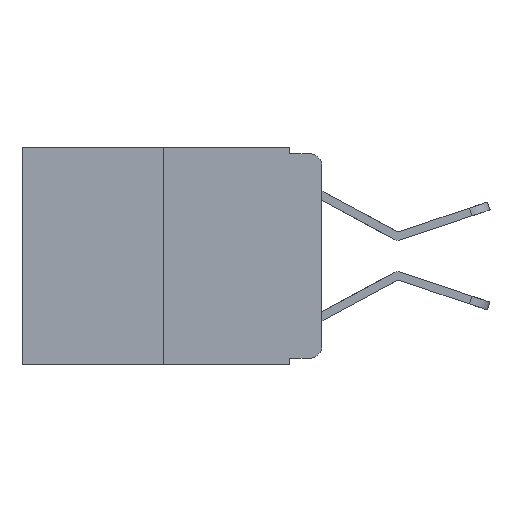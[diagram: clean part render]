
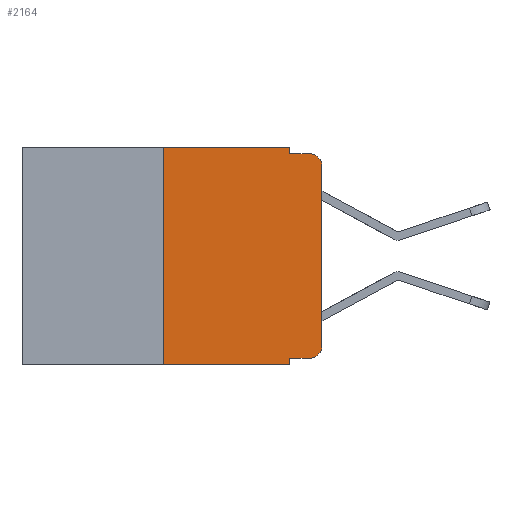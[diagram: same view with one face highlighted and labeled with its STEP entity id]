
A CAD part, left-side view. The second image highlights one B-rep face of the part: STEP entity #2164.
In plain terms, the highlighted planar face has unit normal (-1, 0, 0).
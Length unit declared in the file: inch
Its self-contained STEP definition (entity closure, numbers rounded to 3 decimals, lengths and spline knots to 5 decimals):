
#44 = VERTEX_POINT ( 'NONE', #3486 ) ;
#171 = ORIENTED_EDGE ( 'NONE', *, *, #5372, .F. ) ;
#221 = AXIS2_PLACEMENT_3D ( 'NONE', #3652, #10032, #4606 ) ;
#452 = CARTESIAN_POINT ( 'NONE',  ( 0., 0.473, 0. ) ) ;
#741 = VERTEX_POINT ( 'NONE', #7538 ) ;
#906 = CIRCLE ( 'NONE', #5111, 0.02 ) ;
#935 = CARTESIAN_POINT ( 'NONE',  ( 0., 0.051, -0.333 ) ) ;
#999 = DIRECTION ( 'NONE',  ( 0., 0., -1. ) ) ;
#1063 = EDGE_LOOP ( 'NONE', ( #6013, #10038, #1783, #3662, #11362, #7094, #1661, #171, #7356, #2030 ) ) ;
#1130 = VECTOR ( 'NONE', #10452, 39.37008 ) ;
#1218 = VERTEX_POINT ( 'NONE', #11806 ) ;
#1437 = EDGE_CURVE ( 'NONE', #11429, #4486, #7205, .T. ) ;
#1453 = EDGE_CURVE ( 'NONE', #7406, #8929, #11466, .T. ) ;
#1661 = ORIENTED_EDGE ( 'NONE', *, *, #3476, .T. ) ;
#1755 = DIRECTION ( 'NONE',  ( -1., 0., 0. ) ) ;
#1783 = ORIENTED_EDGE ( 'NONE', *, *, #7295, .F. ) ;
#1883 = DIRECTION ( 'NONE',  ( 0., 0., 1. ) ) ;
#1887 = VECTOR ( 'NONE', #5409, 39.37008 ) ;
#2030 = ORIENTED_EDGE ( 'NONE', *, *, #10388, .T. ) ;
#2081 = EDGE_CURVE ( 'NONE', #44, #1218, #8684, .T. ) ;
#2164 = ADVANCED_FACE ( 'NONE', ( #5705 ), #2243, .F. ) ;
#2243 = PLANE ( 'NONE',  #7349 ) ;
#2609 = CARTESIAN_POINT ( 'NONE',  ( 0., 0.051, 0. ) ) ;
#2661 = CARTESIAN_POINT ( 'NONE',  ( 0., 0.473, 0. ) ) ;
#2714 = VERTEX_POINT ( 'NONE', #8979 ) ;
#2762 = CARTESIAN_POINT ( 'NONE',  ( 0., 0.051, -0.01 ) ) ;
#2818 = LINE ( 'NONE', #10837, #4764 ) ;
#2913 = LINE ( 'NONE', #7643, #9951 ) ;
#3476 = EDGE_CURVE ( 'NONE', #3874, #741, #2818, .T. ) ;
#3486 = CARTESIAN_POINT ( 'NONE',  ( 0., 0.25, 0. ) ) ;
#3596 = LINE ( 'NONE', #10746, #1887 ) ;
#3652 = CARTESIAN_POINT ( 'NONE',  ( 0., 0.02, -0.313 ) ) ;
#3662 = ORIENTED_EDGE ( 'NONE', *, *, #4095, .F. ) ;
#3874 = VERTEX_POINT ( 'NONE', #11005 ) ;
#3882 = CARTESIAN_POINT ( 'NONE',  ( 0., 0., -0.03 ) ) ;
#3947 = LINE ( 'NONE', #11047, #4257 ) ;
#3995 = LINE ( 'NONE', #2609, #6557 ) ;
#4095 = EDGE_CURVE ( 'NONE', #1218, #9621, #3995, .T. ) ;
#4257 = VECTOR ( 'NONE', #1883, 39.37008 ) ;
#4486 = VERTEX_POINT ( 'NONE', #10012 ) ;
#4606 = DIRECTION ( 'NONE',  ( 0., 0., -1. ) ) ;
#4670 = VECTOR ( 'NONE', #6753, 39.37008 ) ;
#4764 = VECTOR ( 'NONE', #11557, 39.37008 ) ;
#5111 = AXIS2_PLACEMENT_3D ( 'NONE', #7523, #1755, #8399 ) ;
#5372 = EDGE_CURVE ( 'NONE', #11429, #741, #2913, .T. ) ;
#5409 = DIRECTION ( 'NONE',  ( 0., -1., 0. ) ) ;
#5580 = CARTESIAN_POINT ( 'NONE',  ( 0., 0., -0.313 ) ) ;
#5705 = FACE_OUTER_BOUND ( 'NONE', #1063, .T. ) ;
#6001 = DIRECTION ( 'NONE',  ( 0., 0., -1. ) ) ;
#6013 = ORIENTED_EDGE ( 'NONE', *, *, #1453, .T. ) ;
#6020 = EDGE_CURVE ( 'NONE', #3874, #44, #3947, .T. ) ;
#6557 = VECTOR ( 'NONE', #999, 39.37008 ) ;
#6607 = CARTESIAN_POINT ( 'NONE',  ( 0., 0.051, -0.333 ) ) ;
#6697 = CARTESIAN_POINT ( 'NONE',  ( 0., 0., 0. ) ) ;
#6727 = DIRECTION ( 'NONE',  ( 0., -1., 0. ) ) ;
#6753 = DIRECTION ( 'NONE',  ( 0., 0., 1. ) ) ;
#6907 = DIRECTION ( 'NONE',  ( 0., 0., -1. ) ) ;
#7094 = ORIENTED_EDGE ( 'NONE', *, *, #6020, .F. ) ;
#7205 = LINE ( 'NONE', #6607, #8319 ) ;
#7295 = EDGE_CURVE ( 'NONE', #9621, #2714, #3596, .T. ) ;
#7349 = AXIS2_PLACEMENT_3D ( 'NONE', #2661, #9963, #6907 ) ;
#7356 = ORIENTED_EDGE ( 'NONE', *, *, #1437, .T. ) ;
#7406 = VERTEX_POINT ( 'NONE', #5580 ) ;
#7523 = CARTESIAN_POINT ( 'NONE',  ( 0., 0.02, -0.03 ) ) ;
#7538 = CARTESIAN_POINT ( 'NONE',  ( 0., 0.051, -0.343 ) ) ;
#7643 = CARTESIAN_POINT ( 'NONE',  ( 0., 0.051, 0. ) ) ;
#8319 = VECTOR ( 'NONE', #6727, 39.37008 ) ;
#8399 = DIRECTION ( 'NONE',  ( 0., 0., -1. ) ) ;
#8684 = LINE ( 'NONE', #452, #1130 ) ;
#8929 = VERTEX_POINT ( 'NONE', #3882 ) ;
#8979 = CARTESIAN_POINT ( 'NONE',  ( 0., 0.02, -0.01 ) ) ;
#9613 = EDGE_CURVE ( 'NONE', #8929, #2714, #906, .T. ) ;
#9621 = VERTEX_POINT ( 'NONE', #2762 ) ;
#9951 = VECTOR ( 'NONE', #6001, 39.37008 ) ;
#9963 = DIRECTION ( 'NONE',  ( 1., 0., 0. ) ) ;
#10012 = CARTESIAN_POINT ( 'NONE',  ( 0., 0.02, -0.333 ) ) ;
#10032 = DIRECTION ( 'NONE',  ( -1., 0., 0. ) ) ;
#10038 = ORIENTED_EDGE ( 'NONE', *, *, #9613, .T. ) ;
#10369 = CIRCLE ( 'NONE', #221, 0.02 ) ;
#10388 = EDGE_CURVE ( 'NONE', #4486, #7406, #10369, .T. ) ;
#10452 = DIRECTION ( 'NONE',  ( 0., -1., 0. ) ) ;
#10746 = CARTESIAN_POINT ( 'NONE',  ( 0., 0.051, -0.01 ) ) ;
#10837 = CARTESIAN_POINT ( 'NONE',  ( 0., 0.473, -0.343 ) ) ;
#11005 = CARTESIAN_POINT ( 'NONE',  ( 0., 0.25, -0.343 ) ) ;
#11047 = CARTESIAN_POINT ( 'NONE',  ( 0., 0.25, 0. ) ) ;
#11362 = ORIENTED_EDGE ( 'NONE', *, *, #2081, .F. ) ;
#11429 = VERTEX_POINT ( 'NONE', #935 ) ;
#11466 = LINE ( 'NONE', #6697, #4670 ) ;
#11557 = DIRECTION ( 'NONE',  ( 0., -1., 0. ) ) ;
#11806 = CARTESIAN_POINT ( 'NONE',  ( 0., 0.051, 0. ) ) ;
